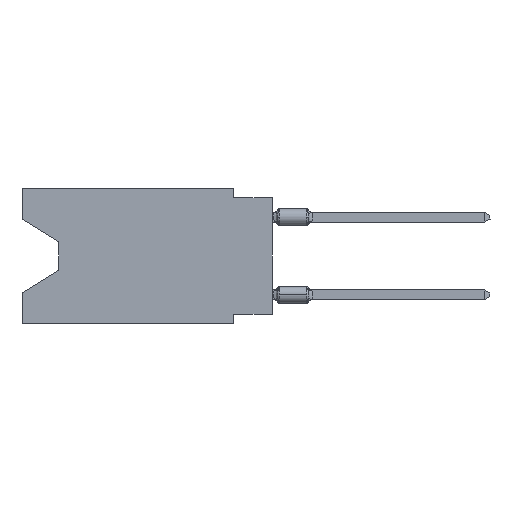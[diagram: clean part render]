
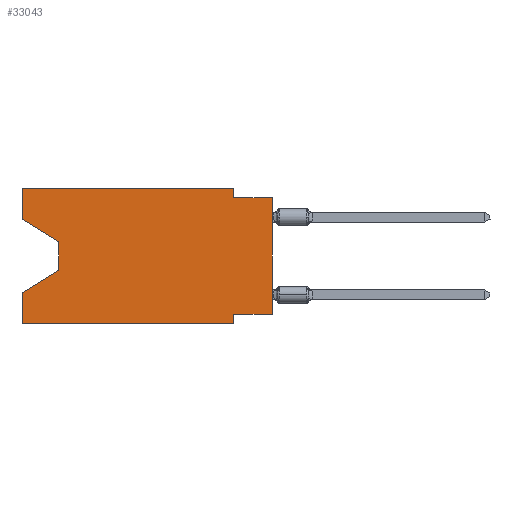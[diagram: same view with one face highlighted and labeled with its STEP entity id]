
A CAD part, left-side view. The second image highlights one B-rep face of the part: STEP entity #33043.
In plain terms, the highlighted planar face has unit normal (-1, 0, 0).
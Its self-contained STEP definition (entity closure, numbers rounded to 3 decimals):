
#1522 = CARTESIAN_POINT ( 'NONE',  ( 0., 0., -0.635 ) ) ;
#1731 = VECTOR ( 'NONE', #11947, 1000. ) ;
#1762 = DIRECTION ( 'NONE',  ( 0., -1., 0. ) ) ;
#3327 = EDGE_CURVE ( 'NONE', #58754, #47589, #22255, .T. ) ;
#3797 = EDGE_CURVE ( 'NONE', #28682, #42920, #12242, .T. ) ;
#4386 = VERTEX_POINT ( 'NONE', #28832 ) ;
#5836 = VERTEX_POINT ( 'NONE', #8554 ) ;
#6467 = EDGE_CURVE ( 'NONE', #49030, #17195, #43789, .T. ) ;
#6481 = EDGE_CURVE ( 'NONE', #42920, #26600, #16741, .T. ) ;
#6954 = EDGE_CURVE ( 'NONE', #35322, #47589, #49914, .T. ) ;
#7412 = DIRECTION ( 'NONE',  ( 0., -1., 0. ) ) ;
#7884 = VECTOR ( 'NONE', #20528, 1000. ) ;
#8554 = CARTESIAN_POINT ( 'NONE',  ( 0., 16.383, 0. ) ) ;
#11910 = CARTESIAN_POINT ( 'NONE',  ( 0., 16.383, 0. ) ) ;
#11947 = DIRECTION ( 'NONE',  ( 0., 0., -1. ) ) ;
#12242 = LINE ( 'NONE', #59504, #1731 ) ;
#12278 = CARTESIAN_POINT ( 'NONE',  ( 0., 0., 0. ) ) ;
#12930 = DIRECTION ( 'NONE',  ( 0., 0., -1. ) ) ;
#12934 = VECTOR ( 'NONE', #40158, 1000. ) ;
#13000 = ORIENTED_EDGE ( 'NONE', *, *, #23951, .T. ) ;
#14391 = VECTOR ( 'NONE', #1762, 1000. ) ;
#14963 = CARTESIAN_POINT ( 'NONE',  ( 0., 0., -0.635 ) ) ;
#15467 = CARTESIAN_POINT ( 'NONE',  ( 0., 16.383, -2.038 ) ) ;
#16741 = LINE ( 'NONE', #1522, #31679 ) ;
#17195 = VERTEX_POINT ( 'NONE', #50881 ) ;
#18161 = VECTOR ( 'NONE', #59242, 1000. ) ;
#19415 = CARTESIAN_POINT ( 'NONE',  ( 0., 16.383, 0. ) ) ;
#20181 = CARTESIAN_POINT ( 'NONE',  ( 0., 13.97, -5.385 ) ) ;
#20528 = DIRECTION ( 'NONE',  ( 0., 0., -1. ) ) ;
#20615 = LINE ( 'NONE', #48901, #12934 ) ;
#20653 = ORIENTED_EDGE ( 'NONE', *, *, #50731, .T. ) ;
#20924 = LINE ( 'NONE', #11910, #44832 ) ;
#21952 = CARTESIAN_POINT ( 'NONE',  ( 0., 2.54, -8.89 ) ) ;
#22255 = LINE ( 'NONE', #21952, #31434 ) ;
#22914 = DIRECTION ( 'NONE',  ( 0., 0., 1. ) ) ;
#23478 = PLANE ( 'NONE',  #29737 ) ;
#23537 = LINE ( 'NONE', #46532, #47496 ) ;
#23951 = EDGE_CURVE ( 'NONE', #42979, #26600, #26887, .T. ) ;
#24644 = CARTESIAN_POINT ( 'NONE',  ( 0., 2.54, 0. ) ) ;
#25274 = LINE ( 'NONE', #54473, #44688 ) ;
#26423 = CARTESIAN_POINT ( 'NONE',  ( 0., 13.97, -3.505 ) ) ;
#26600 = VERTEX_POINT ( 'NONE', #14963 ) ;
#26887 = LINE ( 'NONE', #12278, #43885 ) ;
#28682 = VERTEX_POINT ( 'NONE', #24644 ) ;
#28832 = CARTESIAN_POINT ( 'NONE',  ( 0., 13.97, -3.505 ) ) ;
#29154 = ORIENTED_EDGE ( 'NONE', *, *, #3327, .F. ) ;
#29737 = AXIS2_PLACEMENT_3D ( 'NONE', #19415, #38342, #32786 ) ;
#30856 = DIRECTION ( 'NONE',  ( 0., -1., 0. ) ) ;
#31240 = ORIENTED_EDGE ( 'NONE', *, *, #6481, .F. ) ;
#31434 = VECTOR ( 'NONE', #12930, 1000. ) ;
#31679 = VECTOR ( 'NONE', #7412, 1000. ) ;
#31816 = CARTESIAN_POINT ( 'NONE',  ( 0., 0., -8.255 ) ) ;
#32786 = DIRECTION ( 'NONE',  ( 0., 0., -1. ) ) ;
#33013 = CARTESIAN_POINT ( 'NONE',  ( 0., 2.54, -8.255 ) ) ;
#33043 = ADVANCED_FACE ( 'NONE', ( #57667 ), #23478, .F. ) ;
#35322 = VERTEX_POINT ( 'NONE', #41580 ) ;
#35934 = ORIENTED_EDGE ( 'NONE', *, *, #47910, .F. ) ;
#36049 = EDGE_CURVE ( 'NONE', #42979, #58754, #25274, .T. ) ;
#38342 = DIRECTION ( 'NONE',  ( 1., 0., 0. ) ) ;
#38504 = VERTEX_POINT ( 'NONE', #15467 ) ;
#40158 = DIRECTION ( 'NONE',  ( 0., -0.855, -0.519 ) ) ;
#40565 = CARTESIAN_POINT ( 'NONE',  ( 0., 16.383, -8.89 ) ) ;
#41125 = ORIENTED_EDGE ( 'NONE', *, *, #36049, .F. ) ;
#41580 = CARTESIAN_POINT ( 'NONE',  ( 0., 16.383, -8.89 ) ) ;
#42920 = VERTEX_POINT ( 'NONE', #59203 ) ;
#42979 = VERTEX_POINT ( 'NONE', #31816 ) ;
#43106 = ORIENTED_EDGE ( 'NONE', *, *, #56942, .F. ) ;
#43789 = LINE ( 'NONE', #20181, #57492 ) ;
#43885 = VECTOR ( 'NONE', #45831, 1000. ) ;
#44688 = VECTOR ( 'NONE', #49488, 1000. ) ;
#44832 = VECTOR ( 'NONE', #30856, 1000. ) ;
#45831 = DIRECTION ( 'NONE',  ( 0., 0., 1. ) ) ;
#46532 = CARTESIAN_POINT ( 'NONE',  ( 0., 16.383, 0. ) ) ;
#47111 = ORIENTED_EDGE ( 'NONE', *, *, #6954, .T. ) ;
#47496 = VECTOR ( 'NONE', #22914, 1000. ) ;
#47589 = VERTEX_POINT ( 'NONE', #49063 ) ;
#47910 = EDGE_CURVE ( 'NONE', #38504, #5836, #23537, .T. ) ;
#47952 = CARTESIAN_POINT ( 'NONE',  ( 0., 13.97, -5.385 ) ) ;
#48901 = CARTESIAN_POINT ( 'NONE',  ( 0., 16.383, -2.038 ) ) ;
#49030 = VERTEX_POINT ( 'NONE', #47952 ) ;
#49063 = CARTESIAN_POINT ( 'NONE',  ( 0., 2.54, -8.89 ) ) ;
#49362 = ORIENTED_EDGE ( 'NONE', *, *, #3797, .F. ) ;
#49488 = DIRECTION ( 'NONE',  ( 0., 1., 0. ) ) ;
#49914 = LINE ( 'NONE', #40565, #14391 ) ;
#50202 = CARTESIAN_POINT ( 'NONE',  ( 0., 16.383, 0. ) ) ;
#50535 = ORIENTED_EDGE ( 'NONE', *, *, #6467, .T. ) ;
#50731 = EDGE_CURVE ( 'NONE', #4386, #49030, #58775, .T. ) ;
#50881 = CARTESIAN_POINT ( 'NONE',  ( 0., 16.383, -6.852 ) ) ;
#51057 = EDGE_LOOP ( 'NONE', ( #55328, #20653, #50535, #43106, #47111, #29154, #41125, #13000, #31240, #49362, #52973, #35934 ) ) ;
#52004 = EDGE_CURVE ( 'NONE', #38504, #4386, #20615, .T. ) ;
#52973 = ORIENTED_EDGE ( 'NONE', *, *, #53995, .F. ) ;
#53452 = DIRECTION ( 'NONE',  ( 0., 0.855, -0.519 ) ) ;
#53995 = EDGE_CURVE ( 'NONE', #5836, #28682, #20924, .T. ) ;
#54473 = CARTESIAN_POINT ( 'NONE',  ( 0., 0., -8.255 ) ) ;
#55186 = LINE ( 'NONE', #50202, #18161 ) ;
#55328 = ORIENTED_EDGE ( 'NONE', *, *, #52004, .T. ) ;
#56942 = EDGE_CURVE ( 'NONE', #35322, #17195, #55186, .T. ) ;
#57492 = VECTOR ( 'NONE', #53452, 1000. ) ;
#57667 = FACE_OUTER_BOUND ( 'NONE', #51057, .T. ) ;
#58754 = VERTEX_POINT ( 'NONE', #33013 ) ;
#58775 = LINE ( 'NONE', #26423, #7884 ) ;
#59203 = CARTESIAN_POINT ( 'NONE',  ( 0., 2.54, -0.635 ) ) ;
#59242 = DIRECTION ( 'NONE',  ( 0., 0., 1. ) ) ;
#59504 = CARTESIAN_POINT ( 'NONE',  ( 0., 2.54, 0. ) ) ;
